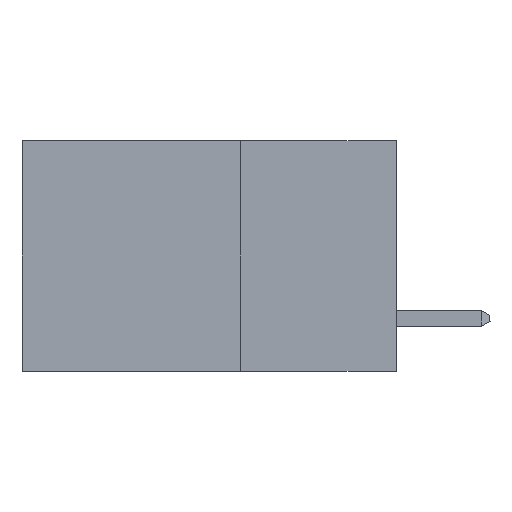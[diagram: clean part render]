
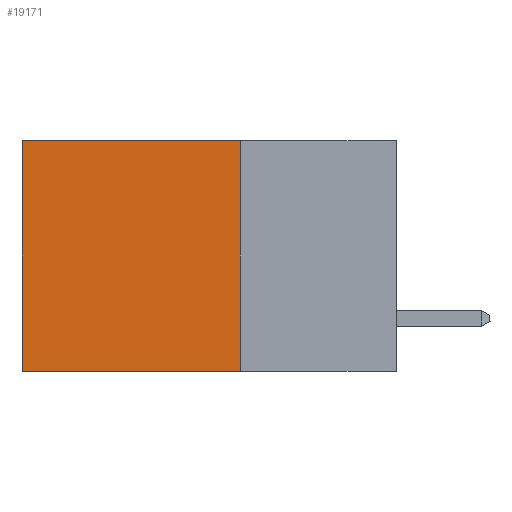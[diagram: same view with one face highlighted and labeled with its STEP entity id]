
A CAD part, left-side view. The second image highlights one B-rep face of the part: STEP entity #19171.
In plain terms, the highlighted planar face has unit normal (-1, 0, 0).
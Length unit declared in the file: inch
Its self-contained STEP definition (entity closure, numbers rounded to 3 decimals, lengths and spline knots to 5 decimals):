
#397 = DIRECTION ( 'NONE',  ( 0., 1., 0. ) ) ;
#1263 = VERTEX_POINT ( 'NONE', #10305 ) ;
#1882 = DIRECTION ( 'NONE',  ( 0., 0., -1. ) ) ;
#2335 = DIRECTION ( 'NONE',  ( 0., 0., -1. ) ) ;
#2470 = CARTESIAN_POINT ( 'NONE',  ( 0.298, 0.25, 0. ) ) ;
#2737 = EDGE_CURVE ( 'NONE', #6166, #20047, #13315, .T. ) ;
#3691 = VECTOR ( 'NONE', #7854, 39.37008 ) ;
#3709 = CARTESIAN_POINT ( 'NONE',  ( 0.298, 0.6, 0. ) ) ;
#3968 = VERTEX_POINT ( 'NONE', #22560 ) ;
#4148 = FACE_OUTER_BOUND ( 'NONE', #19832, .T. ) ;
#4915 = LINE ( 'NONE', #6025, #19191 ) ;
#6025 = CARTESIAN_POINT ( 'NONE',  ( 0.298, 0.25, -0.37 ) ) ;
#6166 = VERTEX_POINT ( 'NONE', #20879 ) ;
#6397 = AXIS2_PLACEMENT_3D ( 'NONE', #21999, #13151, #2335 ) ;
#6538 = CARTESIAN_POINT ( 'NONE',  ( 0.298, 0.25, -0.37 ) ) ;
#7678 = CARTESIAN_POINT ( 'NONE',  ( 0.298, 0.25, 0. ) ) ;
#7854 = DIRECTION ( 'NONE',  ( 0., 0., -1. ) ) ;
#8041 = EDGE_CURVE ( 'NONE', #20047, #3968, #4915, .T. ) ;
#9157 = EDGE_CURVE ( 'NONE', #1263, #3968, #13960, .T. ) ;
#9160 = VECTOR ( 'NONE', #1882, 39.37008 ) ;
#9528 = PLANE ( 'NONE',  #6397 ) ;
#10305 = CARTESIAN_POINT ( 'NONE',  ( 0.298, 0.6, 0. ) ) ;
#12594 = ORIENTED_EDGE ( 'NONE', *, *, #8041, .F. ) ;
#12638 = VECTOR ( 'NONE', #397, 39.37008 ) ;
#13151 = DIRECTION ( 'NONE',  ( 1., 0., 0. ) ) ;
#13315 = LINE ( 'NONE', #2470, #3691 ) ;
#13658 = ORIENTED_EDGE ( 'NONE', *, *, #22895, .T. ) ;
#13960 = LINE ( 'NONE', #3709, #9160 ) ;
#15892 = ORIENTED_EDGE ( 'NONE', *, *, #2737, .F. ) ;
#18161 = ORIENTED_EDGE ( 'NONE', *, *, #9157, .T. ) ;
#18521 = DIRECTION ( 'NONE',  ( 0., 1., 0. ) ) ;
#19171 = ADVANCED_FACE ( 'NONE', ( #4148 ), #9528, .F. ) ;
#19191 = VECTOR ( 'NONE', #18521, 39.37008 ) ;
#19832 = EDGE_LOOP ( 'NONE', ( #18161, #12594, #15892, #13658 ) ) ;
#20047 = VERTEX_POINT ( 'NONE', #6538 ) ;
#20879 = CARTESIAN_POINT ( 'NONE',  ( 0.298, 0.25, 0. ) ) ;
#21535 = LINE ( 'NONE', #7678, #12638 ) ;
#21999 = CARTESIAN_POINT ( 'NONE',  ( 0.298, 0.25, 0. ) ) ;
#22560 = CARTESIAN_POINT ( 'NONE',  ( 0.298, 0.6, -0.37 ) ) ;
#22895 = EDGE_CURVE ( 'NONE', #6166, #1263, #21535, .T. ) ;
